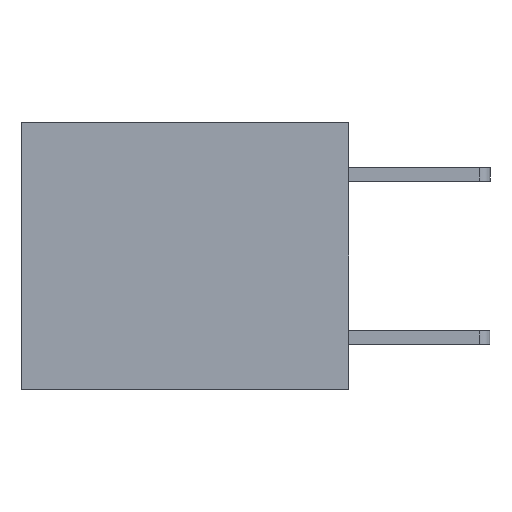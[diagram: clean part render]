
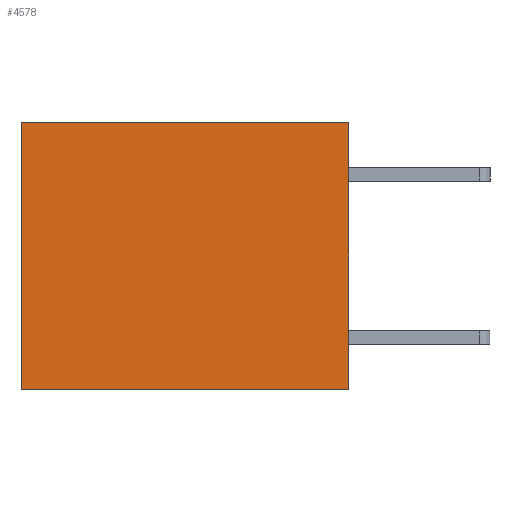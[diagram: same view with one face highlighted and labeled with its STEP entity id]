
A CAD part, left-side view. The second image highlights one B-rep face of the part: STEP entity #4578.
In plain terms, the highlighted planar face has unit normal (-1, 0, 0).
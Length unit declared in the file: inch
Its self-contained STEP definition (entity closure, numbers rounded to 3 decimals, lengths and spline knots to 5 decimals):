
#277 = CARTESIAN_POINT ( 'NONE',  ( 0.3165, 0., -0.49 ) ) ;
#476 = DIRECTION ( 'NONE',  ( 0., 0., -1. ) ) ;
#547 = CARTESIAN_POINT ( 'NONE',  ( 0.3165, 0., -0.49 ) ) ;
#614 = CARTESIAN_POINT ( 'NONE',  ( 0.3165, 0., 0. ) ) ;
#813 = VERTEX_POINT ( 'NONE', #11218 ) ;
#1408 = DIRECTION ( 'NONE',  ( 0., 0., -1. ) ) ;
#1997 = VECTOR ( 'NONE', #3942, 39.37008 ) ;
#2530 = VERTEX_POINT ( 'NONE', #6491 ) ;
#2592 = VECTOR ( 'NONE', #6641, 39.37008 ) ;
#3899 = FACE_OUTER_BOUND ( 'NONE', #5439, .T. ) ;
#3942 = DIRECTION ( 'NONE',  ( 0., 1., 0. ) ) ;
#4035 = EDGE_CURVE ( 'NONE', #813, #8362, #7770, .T. ) ;
#4347 = CARTESIAN_POINT ( 'NONE',  ( 0.3165, 0., -0.49 ) ) ;
#4578 = ADVANCED_FACE ( 'NONE', ( #3899 ), #7461, .F. ) ;
#4742 = ORIENTED_EDGE ( 'NONE', *, *, #7708, .F. ) ;
#5084 = ORIENTED_EDGE ( 'NONE', *, *, #5367, .T. ) ;
#5160 = LINE ( 'NONE', #277, #2592 ) ;
#5367 = EDGE_CURVE ( 'NONE', #7171, #813, #9236, .T. ) ;
#5396 = ORIENTED_EDGE ( 'NONE', *, *, #4035, .T. ) ;
#5439 = EDGE_LOOP ( 'NONE', ( #5396, #4742, #5500, #5084 ) ) ;
#5500 = ORIENTED_EDGE ( 'NONE', *, *, #7917, .F. ) ;
#6044 = AXIS2_PLACEMENT_3D ( 'NONE', #547, #6631, #1408 ) ;
#6491 = CARTESIAN_POINT ( 'NONE',  ( 0.3165, 0., -0.49 ) ) ;
#6631 = DIRECTION ( 'NONE',  ( 1., 0., 0. ) ) ;
#6641 = DIRECTION ( 'NONE',  ( 0., 1., 0. ) ) ;
#6952 = CARTESIAN_POINT ( 'NONE',  ( 0.3165, 0.6, -0.49 ) ) ;
#7171 = VERTEX_POINT ( 'NONE', #11168 ) ;
#7461 = PLANE ( 'NONE',  #6044 ) ;
#7708 = EDGE_CURVE ( 'NONE', #2530, #8362, #5160, .T. ) ;
#7770 = LINE ( 'NONE', #8439, #8165 ) ;
#7917 = EDGE_CURVE ( 'NONE', #7171, #2530, #10649, .T. ) ;
#8165 = VECTOR ( 'NONE', #476, 39.37008 ) ;
#8362 = VERTEX_POINT ( 'NONE', #6952 ) ;
#8439 = CARTESIAN_POINT ( 'NONE',  ( 0.3165, 0.6, -0.49 ) ) ;
#9236 = LINE ( 'NONE', #614, #1997 ) ;
#10092 = VECTOR ( 'NONE', #10482, 39.37008 ) ;
#10482 = DIRECTION ( 'NONE',  ( 0., 0., -1. ) ) ;
#10649 = LINE ( 'NONE', #4347, #10092 ) ;
#11168 = CARTESIAN_POINT ( 'NONE',  ( 0.3165, 0., 0. ) ) ;
#11218 = CARTESIAN_POINT ( 'NONE',  ( 0.3165, 0.6, 0. ) ) ;
